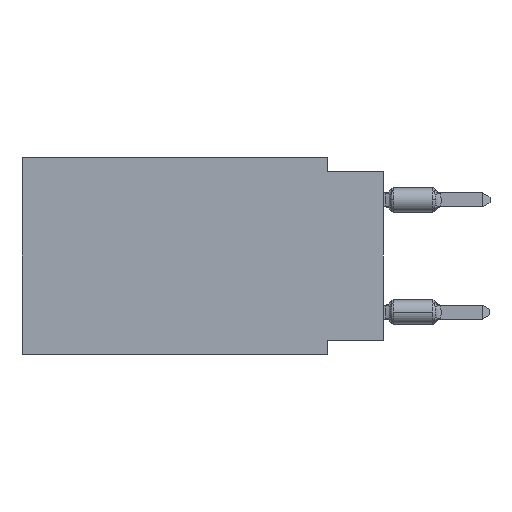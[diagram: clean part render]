
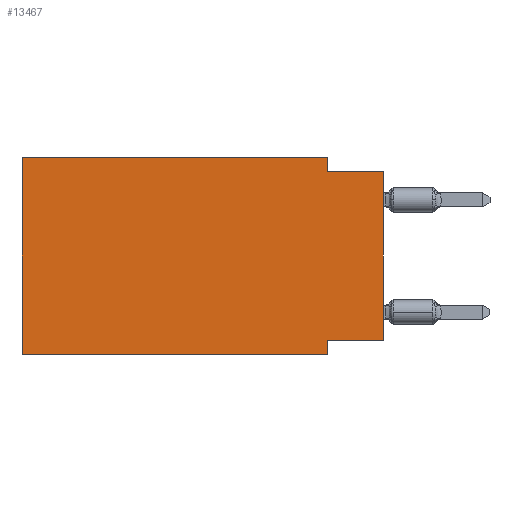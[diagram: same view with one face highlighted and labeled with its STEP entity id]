
A CAD part, left-side view. The second image highlights one B-rep face of the part: STEP entity #13467.
In plain terms, the highlighted planar face has unit normal (-1, 0, 0).
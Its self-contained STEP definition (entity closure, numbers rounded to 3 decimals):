
#32 = LINE ( 'NONE', #3267, #10264 ) ;
#583 = CARTESIAN_POINT ( 'NONE',  ( 0., 0., 0. ) ) ;
#808 = LINE ( 'NONE', #19309, #17294 ) ;
#1988 = DIRECTION ( 'NONE',  ( 1., 0., 0. ) ) ;
#2015 = ORIENTED_EDGE ( 'NONE', *, *, #18982, .F. ) ;
#2118 = CARTESIAN_POINT ( 'NONE',  ( 0., 16.383, -8.89 ) ) ;
#2181 = CARTESIAN_POINT ( 'NONE',  ( 0., 2.54, 0. ) ) ;
#2366 = VERTEX_POINT ( 'NONE', #5586 ) ;
#2471 = EDGE_CURVE ( 'NONE', #16782, #12380, #15275, .T. ) ;
#2488 = ORIENTED_EDGE ( 'NONE', *, *, #8718, .T. ) ;
#2529 = CARTESIAN_POINT ( 'NONE',  ( 0., 0., -0.635 ) ) ;
#3061 = VECTOR ( 'NONE', #6746, 1000. ) ;
#3170 = VECTOR ( 'NONE', #3467, 1000. ) ;
#3267 = CARTESIAN_POINT ( 'NONE',  ( 0., 2.54, -8.89 ) ) ;
#3425 = EDGE_CURVE ( 'NONE', #12380, #18758, #12533, .T. ) ;
#3467 = DIRECTION ( 'NONE',  ( 0., -1., 0. ) ) ;
#3772 = EDGE_LOOP ( 'NONE', ( #16899, #2015, #10772, #18104, #6178, #2488, #13982, #13172 ) ) ;
#4321 = CARTESIAN_POINT ( 'NONE',  ( 0., 2.54, -8.89 ) ) ;
#4614 = DIRECTION ( 'NONE',  ( 0., 0., 1. ) ) ;
#5456 = DIRECTION ( 'NONE',  ( 0., -1., 0. ) ) ;
#5586 = CARTESIAN_POINT ( 'NONE',  ( 0., 0., -8.255 ) ) ;
#5888 = CARTESIAN_POINT ( 'NONE',  ( 0., 16.383, 0. ) ) ;
#5943 = CARTESIAN_POINT ( 'NONE',  ( 0., 2.54, 0. ) ) ;
#6178 = ORIENTED_EDGE ( 'NONE', *, *, #10416, .F. ) ;
#6500 = CARTESIAN_POINT ( 'NONE',  ( 0., 2.54, -0.635 ) ) ;
#6746 = DIRECTION ( 'NONE',  ( 0., 0., 1. ) ) ;
#7418 = EDGE_CURVE ( 'NONE', #2366, #18690, #12628, .T. ) ;
#7863 = DIRECTION ( 'NONE',  ( 0., 1., 0. ) ) ;
#8289 = VECTOR ( 'NONE', #7863, 1000. ) ;
#8718 = EDGE_CURVE ( 'NONE', #16421, #8789, #808, .T. ) ;
#8789 = VERTEX_POINT ( 'NONE', #4321 ) ;
#8927 = VECTOR ( 'NONE', #12059, 1000. ) ;
#8990 = EDGE_CURVE ( 'NONE', #2366, #19331, #9302, .T. ) ;
#9302 = LINE ( 'NONE', #12430, #8289 ) ;
#10264 = VECTOR ( 'NONE', #14075, 1000. ) ;
#10416 = EDGE_CURVE ( 'NONE', #16421, #16782, #11637, .T. ) ;
#10772 = ORIENTED_EDGE ( 'NONE', *, *, #3425, .F. ) ;
#11149 = LINE ( 'NONE', #2529, #3170 ) ;
#11288 = FACE_OUTER_BOUND ( 'NONE', #3772, .T. ) ;
#11637 = LINE ( 'NONE', #18370, #19294 ) ;
#12059 = DIRECTION ( 'NONE',  ( 0., -1., 0. ) ) ;
#12380 = VERTEX_POINT ( 'NONE', #2181 ) ;
#12430 = CARTESIAN_POINT ( 'NONE',  ( 0., 0., -8.255 ) ) ;
#12533 = LINE ( 'NONE', #5943, #14443 ) ;
#12628 = LINE ( 'NONE', #583, #3061 ) ;
#12932 = CARTESIAN_POINT ( 'NONE',  ( 0., 2.54, -8.255 ) ) ;
#13172 = ORIENTED_EDGE ( 'NONE', *, *, #8990, .F. ) ;
#13467 = ADVANCED_FACE ( 'NONE', ( #11288 ), #15918, .F. ) ;
#13982 = ORIENTED_EDGE ( 'NONE', *, *, #18737, .F. ) ;
#14075 = DIRECTION ( 'NONE',  ( 0., 0., -1. ) ) ;
#14307 = DIRECTION ( 'NONE',  ( 0., 0., -1. ) ) ;
#14443 = VECTOR ( 'NONE', #15331, 1000. ) ;
#15275 = LINE ( 'NONE', #5888, #8927 ) ;
#15331 = DIRECTION ( 'NONE',  ( 0., 0., -1. ) ) ;
#15443 = CARTESIAN_POINT ( 'NONE',  ( 0., 16.383, 0. ) ) ;
#15831 = CARTESIAN_POINT ( 'NONE',  ( 0., 16.383, 0. ) ) ;
#15918 = PLANE ( 'NONE',  #16983 ) ;
#16421 = VERTEX_POINT ( 'NONE', #2118 ) ;
#16782 = VERTEX_POINT ( 'NONE', #15443 ) ;
#16899 = ORIENTED_EDGE ( 'NONE', *, *, #7418, .T. ) ;
#16983 = AXIS2_PLACEMENT_3D ( 'NONE', #15831, #1988, #14307 ) ;
#17294 = VECTOR ( 'NONE', #5456, 1000. ) ;
#18104 = ORIENTED_EDGE ( 'NONE', *, *, #2471, .F. ) ;
#18370 = CARTESIAN_POINT ( 'NONE',  ( 0., 16.383, 0. ) ) ;
#18690 = VERTEX_POINT ( 'NONE', #19835 ) ;
#18737 = EDGE_CURVE ( 'NONE', #19331, #8789, #32, .T. ) ;
#18758 = VERTEX_POINT ( 'NONE', #6500 ) ;
#18982 = EDGE_CURVE ( 'NONE', #18758, #18690, #11149, .T. ) ;
#19294 = VECTOR ( 'NONE', #4614, 1000. ) ;
#19309 = CARTESIAN_POINT ( 'NONE',  ( 0., 16.383, -8.89 ) ) ;
#19331 = VERTEX_POINT ( 'NONE', #12932 ) ;
#19835 = CARTESIAN_POINT ( 'NONE',  ( 0., 0., -0.635 ) ) ;
